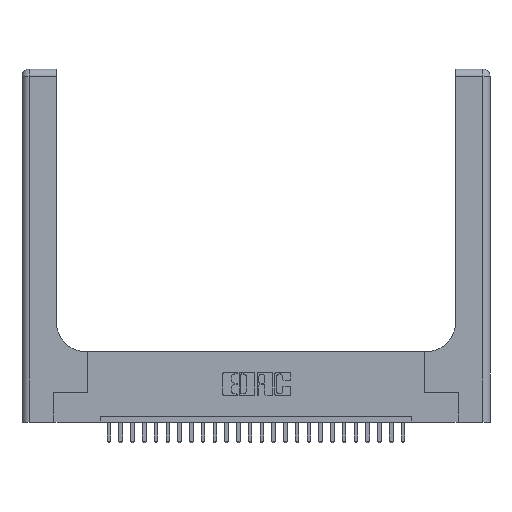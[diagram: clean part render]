
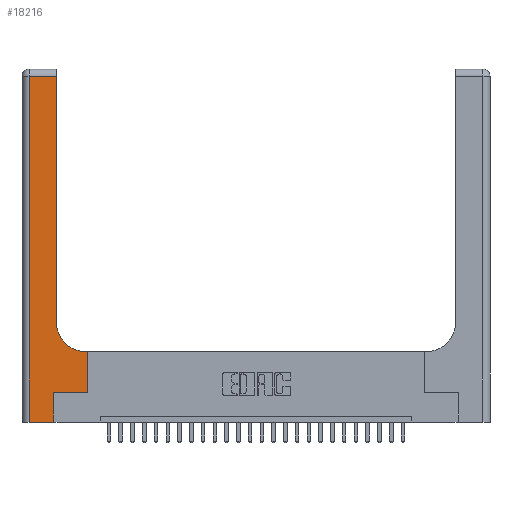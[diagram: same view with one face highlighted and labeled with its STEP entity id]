
A CAD part, top view. The second image highlights one B-rep face of the part: STEP entity #18216.
In plain terms, the highlighted planar face has unit normal (0, 0, 1).
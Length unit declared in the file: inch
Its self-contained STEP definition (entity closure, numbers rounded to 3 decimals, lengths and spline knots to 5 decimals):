
#170 = VECTOR ( 'NONE', #13323, 39.37008 ) ;
#446 = DIRECTION ( 'NONE',  ( 0., -1., 0. ) ) ;
#742 = DIRECTION ( 'NONE',  ( -1., 0., 0. ) ) ;
#1070 = CARTESIAN_POINT ( 'NONE',  ( 0.06, 0., 0.37 ) ) ;
#1780 = DIRECTION ( 'NONE',  ( 0., 0., -1. ) ) ;
#2301 = ORIENTED_EDGE ( 'NONE', *, *, #16566, .T. ) ;
#2560 = CARTESIAN_POINT ( 'NONE',  ( 0., 2.94, 0.37 ) ) ;
#2927 = CIRCLE ( 'NONE', #26189, 0.25 ) ;
#2988 = CARTESIAN_POINT ( 'NONE',  ( 0.06, 2.94, 0.37 ) ) ;
#3269 = CARTESIAN_POINT ( 'NONE',  ( 0.5415, 0.6, 0.37 ) ) ;
#3467 = LINE ( 'NONE', #13168, #5422 ) ;
#3720 = EDGE_CURVE ( 'NONE', #16005, #18100, #8410, .T. ) ;
#4578 = VERTEX_POINT ( 'NONE', #3269 ) ;
#5107 = CARTESIAN_POINT ( 'NONE',  ( 0.5585, 0.25, 0.37 ) ) ;
#5110 = AXIS2_PLACEMENT_3D ( 'NONE', #9721, #16052, #26545 ) ;
#5422 = VECTOR ( 'NONE', #742, 39.37008 ) ;
#5753 = CARTESIAN_POINT ( 'NONE',  ( 0.269, 0.25, 0.37 ) ) ;
#5891 = CARTESIAN_POINT ( 'NONE',  ( 0.5415, 0.85, 0.37 ) ) ;
#6051 = VERTEX_POINT ( 'NONE', #13462 ) ;
#6285 = VERTEX_POINT ( 'NONE', #9223 ) ;
#6493 = ORIENTED_EDGE ( 'NONE', *, *, #25944, .T. ) ;
#7036 = LINE ( 'NONE', #11498, #170 ) ;
#7989 = LINE ( 'NONE', #25422, #18393 ) ;
#8324 = VECTOR ( 'NONE', #17625, 39.37008 ) ;
#8410 = LINE ( 'NONE', #5107, #14587 ) ;
#8536 = ORIENTED_EDGE ( 'NONE', *, *, #23236, .T. ) ;
#9223 = CARTESIAN_POINT ( 'NONE',  ( 0.2915, 0.85, 0.37 ) ) ;
#9359 = VECTOR ( 'NONE', #17550, 39.37008 ) ;
#9721 = CARTESIAN_POINT ( 'NONE',  ( 0., 3., 0.37 ) ) ;
#9954 = EDGE_CURVE ( 'NONE', #17493, #13548, #7036, .T. ) ;
#10141 = VECTOR ( 'NONE', #22487, 39.37008 ) ;
#10409 = CARTESIAN_POINT ( 'NONE',  ( 0.5585, 0.25, 0.37 ) ) ;
#10755 = VERTEX_POINT ( 'NONE', #2988 ) ;
#11498 = CARTESIAN_POINT ( 'NONE',  ( 0., 0., 0.37 ) ) ;
#11978 = VERTEX_POINT ( 'NONE', #5753 ) ;
#12293 = LINE ( 'NONE', #19554, #9359 ) ;
#13078 = CARTESIAN_POINT ( 'NONE',  ( 0.269, 0., 0.37 ) ) ;
#13168 = CARTESIAN_POINT ( 'NONE',  ( 0.2915, 0.6, 0.37 ) ) ;
#13203 = EDGE_CURVE ( 'NONE', #6285, #6051, #13400, .T. ) ;
#13323 = DIRECTION ( 'NONE',  ( 1., 0., 0. ) ) ;
#13325 = LINE ( 'NONE', #2560, #21145 ) ;
#13400 = LINE ( 'NONE', #26358, #10141 ) ;
#13462 = CARTESIAN_POINT ( 'NONE',  ( 0.2915, 2.94, 0.37 ) ) ;
#13548 = VERTEX_POINT ( 'NONE', #13078 ) ;
#13965 = PLANE ( 'NONE',  #5110 ) ;
#14587 = VECTOR ( 'NONE', #18166, 39.37008 ) ;
#15597 = CARTESIAN_POINT ( 'NONE',  ( 0.269, 0.25, 0.37 ) ) ;
#16005 = VERTEX_POINT ( 'NONE', #10409 ) ;
#16052 = DIRECTION ( 'NONE',  ( 0., 0., -1. ) ) ;
#16432 = DIRECTION ( 'NONE',  ( 1., 0., 0. ) ) ;
#16566 = EDGE_CURVE ( 'NONE', #4578, #6285, #2927, .T. ) ;
#17493 = VERTEX_POINT ( 'NONE', #1070 ) ;
#17550 = DIRECTION ( 'NONE',  ( 0., 1., 0. ) ) ;
#17625 = DIRECTION ( 'NONE',  ( 1., 0., 0. ) ) ;
#17720 = ORIENTED_EDGE ( 'NONE', *, *, #18050, .T. ) ;
#18050 = EDGE_CURVE ( 'NONE', #13548, #11978, #12293, .T. ) ;
#18066 = LINE ( 'NONE', #15597, #8324 ) ;
#18100 = VERTEX_POINT ( 'NONE', #23815 ) ;
#18166 = DIRECTION ( 'NONE',  ( 0., 1., 0. ) ) ;
#18216 = ADVANCED_FACE ( 'NONE', ( #21709 ), #13965, .F. ) ;
#18393 = VECTOR ( 'NONE', #446, 39.37008 ) ;
#18649 = ORIENTED_EDGE ( 'NONE', *, *, #3720, .T. ) ;
#19148 = EDGE_CURVE ( 'NONE', #10755, #17493, #7989, .T. ) ;
#19303 = DIRECTION ( 'NONE',  ( -1., 0., 0. ) ) ;
#19554 = CARTESIAN_POINT ( 'NONE',  ( 0.269, 0., 0.37 ) ) ;
#20662 = EDGE_LOOP ( 'NONE', ( #21285, #8536, #21880, #22959, #17720, #6493, #18649, #24108, #2301 ) ) ;
#21145 = VECTOR ( 'NONE', #19303, 39.37008 ) ;
#21285 = ORIENTED_EDGE ( 'NONE', *, *, #13203, .T. ) ;
#21709 = FACE_OUTER_BOUND ( 'NONE', #20662, .T. ) ;
#21880 = ORIENTED_EDGE ( 'NONE', *, *, #19148, .T. ) ;
#22487 = DIRECTION ( 'NONE',  ( 0., 1., 0. ) ) ;
#22959 = ORIENTED_EDGE ( 'NONE', *, *, #9954, .T. ) ;
#23236 = EDGE_CURVE ( 'NONE', #6051, #10755, #13325, .T. ) ;
#23815 = CARTESIAN_POINT ( 'NONE',  ( 0.5585, 0.6, 0.37 ) ) ;
#24108 = ORIENTED_EDGE ( 'NONE', *, *, #24478, .T. ) ;
#24478 = EDGE_CURVE ( 'NONE', #18100, #4578, #3467, .T. ) ;
#25422 = CARTESIAN_POINT ( 'NONE',  ( 0.06, 3., 0.37 ) ) ;
#25944 = EDGE_CURVE ( 'NONE', #11978, #16005, #18066, .T. ) ;
#26189 = AXIS2_PLACEMENT_3D ( 'NONE', #5891, #1780, #16432 ) ;
#26358 = CARTESIAN_POINT ( 'NONE',  ( 0.2915, 3., 0.37 ) ) ;
#26545 = DIRECTION ( 'NONE',  ( -1., 0., 0. ) ) ;
